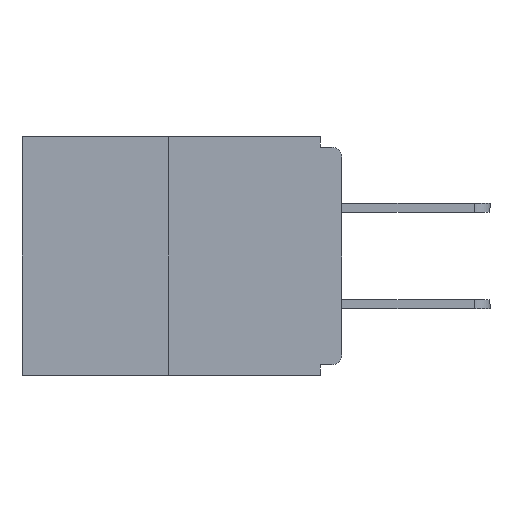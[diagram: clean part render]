
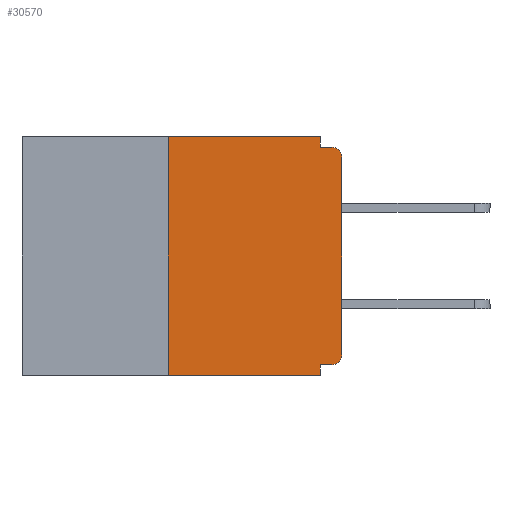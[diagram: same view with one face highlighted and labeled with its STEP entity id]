
A CAD part, left-side view. The second image highlights one B-rep face of the part: STEP entity #30570.
In plain terms, the highlighted planar face has unit normal (-1, 0, 0).
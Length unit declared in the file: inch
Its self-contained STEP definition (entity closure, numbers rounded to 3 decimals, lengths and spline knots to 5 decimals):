
#845 = CARTESIAN_POINT ( 'NONE',  ( 0., 0.46, -0.343 ) ) ;
#1151 = LINE ( 'NONE', #13656, #9465 ) ;
#1425 = CARTESIAN_POINT ( 'NONE',  ( 0., 0.031, -0.343 ) ) ;
#1435 = EDGE_CURVE ( 'NONE', #9978, #9108, #28832, .T. ) ;
#1855 = CARTESIAN_POINT ( 'NONE',  ( 0., 0., -0.015 ) ) ;
#2366 = VERTEX_POINT ( 'NONE', #1425 ) ;
#2713 = VECTOR ( 'NONE', #15898, 39.37008 ) ;
#3469 = VECTOR ( 'NONE', #16095, 39.37008 ) ;
#3724 = EDGE_LOOP ( 'NONE', ( #19290, #10896, #26615, #21875, #26842, #6441, #5229, #21814, #14210, #11633 ) ) ;
#4189 = VERTEX_POINT ( 'NONE', #8218 ) ;
#4869 = CARTESIAN_POINT ( 'NONE',  ( 0., 0.015, -0.03 ) ) ;
#5156 = VERTEX_POINT ( 'NONE', #23916 ) ;
#5229 = ORIENTED_EDGE ( 'NONE', *, *, #7151, .T. ) ;
#5321 = CIRCLE ( 'NONE', #15476, 0.015 ) ;
#5325 = PLANE ( 'NONE',  #27160 ) ;
#5340 = LINE ( 'NONE', #845, #23805 ) ;
#5363 = LINE ( 'NONE', #23025, #3469 ) ;
#5492 = EDGE_CURVE ( 'NONE', #16177, #2366, #18061, .T. ) ;
#5623 = EDGE_CURVE ( 'NONE', #17094, #9108, #16205, .T. ) ;
#6441 = ORIENTED_EDGE ( 'NONE', *, *, #29333, .T. ) ;
#6492 = CARTESIAN_POINT ( 'NONE',  ( 0., 0.031, -0.343 ) ) ;
#6507 = VERTEX_POINT ( 'NONE', #23658 ) ;
#7151 = EDGE_CURVE ( 'NONE', #4189, #17094, #13462, .T. ) ;
#7343 = DIRECTION ( 'NONE',  ( -1., 0., 0. ) ) ;
#7631 = DIRECTION ( 'NONE',  ( 0., 0., 1. ) ) ;
#8174 = FACE_OUTER_BOUND ( 'NONE', #3724, .T. ) ;
#8218 = CARTESIAN_POINT ( 'NONE',  ( 0., 0., -0.313 ) ) ;
#9108 = VERTEX_POINT ( 'NONE', #23071 ) ;
#9260 = DIRECTION ( 'NONE',  ( 0., 0., -1. ) ) ;
#9440 = DIRECTION ( 'NONE',  ( -1., 0., 0. ) ) ;
#9465 = VECTOR ( 'NONE', #9260, 39.37008 ) ;
#9978 = VERTEX_POINT ( 'NONE', #15784 ) ;
#10608 = AXIS2_PLACEMENT_3D ( 'NONE', #4869, #7343, #21479 ) ;
#10896 = ORIENTED_EDGE ( 'NONE', *, *, #23468, .F. ) ;
#11095 = EDGE_CURVE ( 'NONE', #5156, #2366, #5340, .T. ) ;
#11633 = ORIENTED_EDGE ( 'NONE', *, *, #14814, .F. ) ;
#11804 = DIRECTION ( 'NONE',  ( 0., -1., 0. ) ) ;
#11985 = VECTOR ( 'NONE', #7631, 39.37008 ) ;
#13282 = CARTESIAN_POINT ( 'NONE',  ( 0., 0.031, -0.328 ) ) ;
#13462 = LINE ( 'NONE', #26247, #11985 ) ;
#13490 = CARTESIAN_POINT ( 'NONE',  ( 0., 0.46, 0. ) ) ;
#13656 = CARTESIAN_POINT ( 'NONE',  ( 0., 0.031, 0. ) ) ;
#14210 = ORIENTED_EDGE ( 'NONE', *, *, #1435, .F. ) ;
#14814 = EDGE_CURVE ( 'NONE', #6507, #9978, #1151, .T. ) ;
#15027 = CARTESIAN_POINT ( 'NONE',  ( 0., 0.46, 0. ) ) ;
#15447 = VECTOR ( 'NONE', #28046, 39.37008 ) ;
#15476 = AXIS2_PLACEMENT_3D ( 'NONE', #28584, #9440, #30980 ) ;
#15588 = EDGE_CURVE ( 'NONE', #21347, #16177, #27839, .T. ) ;
#15784 = CARTESIAN_POINT ( 'NONE',  ( 0., 0.031, -0.015 ) ) ;
#15898 = DIRECTION ( 'NONE',  ( 0., -1., 0. ) ) ;
#16095 = DIRECTION ( 'NONE',  ( 0., 0., 1. ) ) ;
#16176 = DIRECTION ( 'NONE',  ( 0., -1., 0. ) ) ;
#16177 = VERTEX_POINT ( 'NONE', #13282 ) ;
#16205 = CIRCLE ( 'NONE', #10608, 0.015 ) ;
#16286 = LINE ( 'NONE', #13490, #2713 ) ;
#17026 = CARTESIAN_POINT ( 'NONE',  ( 0., 0.015, -0.328 ) ) ;
#17094 = VERTEX_POINT ( 'NONE', #21398 ) ;
#17413 = DIRECTION ( 'NONE',  ( 0., 0., -1. ) ) ;
#18061 = LINE ( 'NONE', #6492, #15447 ) ;
#19290 = ORIENTED_EDGE ( 'NONE', *, *, #28803, .F. ) ;
#19906 = VECTOR ( 'NONE', #25649, 39.37008 ) ;
#21347 = VERTEX_POINT ( 'NONE', #17026 ) ;
#21398 = CARTESIAN_POINT ( 'NONE',  ( 0., 0., -0.03 ) ) ;
#21479 = DIRECTION ( 'NONE',  ( 0., 0., -1. ) ) ;
#21814 = ORIENTED_EDGE ( 'NONE', *, *, #5623, .T. ) ;
#21875 = ORIENTED_EDGE ( 'NONE', *, *, #5492, .F. ) ;
#23025 = CARTESIAN_POINT ( 'NONE',  ( 0., 0.25, 0. ) ) ;
#23071 = CARTESIAN_POINT ( 'NONE',  ( 0., 0.015, -0.015 ) ) ;
#23468 = EDGE_CURVE ( 'NONE', #5156, #23933, #5363, .T. ) ;
#23658 = CARTESIAN_POINT ( 'NONE',  ( 0., 0.031, 0. ) ) ;
#23805 = VECTOR ( 'NONE', #11804, 39.37008 ) ;
#23916 = CARTESIAN_POINT ( 'NONE',  ( 0., 0.25, -0.343 ) ) ;
#23933 = VERTEX_POINT ( 'NONE', #24597 ) ;
#24597 = CARTESIAN_POINT ( 'NONE',  ( 0., 0.25, 0. ) ) ;
#24799 = DIRECTION ( 'NONE',  ( 1., 0., 0. ) ) ;
#25547 = CARTESIAN_POINT ( 'NONE',  ( 0., 0., -0.328 ) ) ;
#25649 = DIRECTION ( 'NONE',  ( 0., 1., 0. ) ) ;
#26247 = CARTESIAN_POINT ( 'NONE',  ( 0., 0., 0. ) ) ;
#26535 = VECTOR ( 'NONE', #16176, 39.37008 ) ;
#26615 = ORIENTED_EDGE ( 'NONE', *, *, #11095, .T. ) ;
#26842 = ORIENTED_EDGE ( 'NONE', *, *, #15588, .F. ) ;
#27160 = AXIS2_PLACEMENT_3D ( 'NONE', #15027, #24799, #17413 ) ;
#27839 = LINE ( 'NONE', #25547, #19906 ) ;
#28046 = DIRECTION ( 'NONE',  ( 0., 0., -1. ) ) ;
#28584 = CARTESIAN_POINT ( 'NONE',  ( 0., 0.015, -0.313 ) ) ;
#28803 = EDGE_CURVE ( 'NONE', #23933, #6507, #16286, .T. ) ;
#28832 = LINE ( 'NONE', #1855, #26535 ) ;
#29333 = EDGE_CURVE ( 'NONE', #21347, #4189, #5321, .T. ) ;
#30570 = ADVANCED_FACE ( 'NONE', ( #8174 ), #5325, .F. ) ;
#30980 = DIRECTION ( 'NONE',  ( 0., 0., -1. ) ) ;
